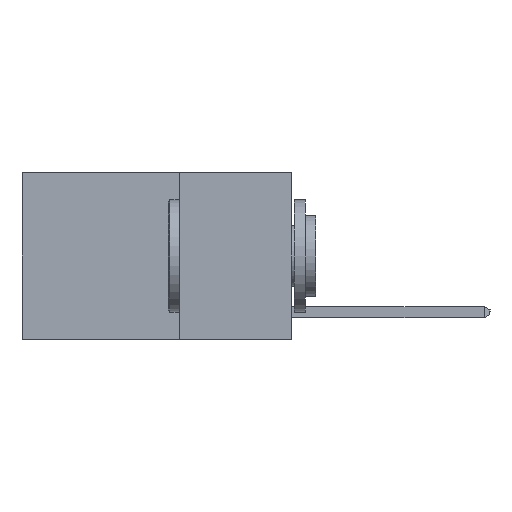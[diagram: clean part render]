
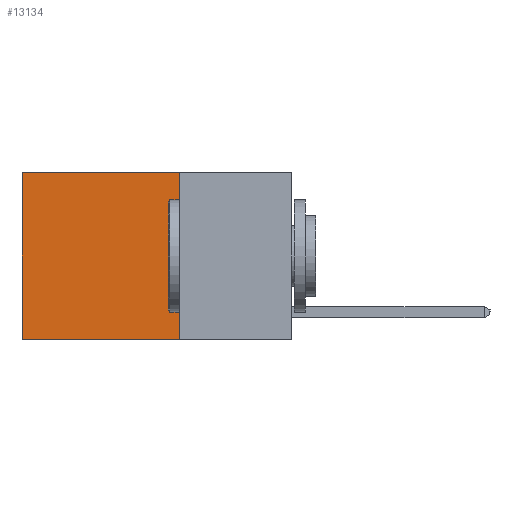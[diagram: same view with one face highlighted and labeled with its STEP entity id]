
A CAD part, left-side view. The second image highlights one B-rep face of the part: STEP entity #13134.
In plain terms, the highlighted planar face has unit normal (-1, 0, 0).
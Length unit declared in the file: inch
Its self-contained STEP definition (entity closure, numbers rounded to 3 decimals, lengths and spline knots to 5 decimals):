
#65 = VERTEX_POINT ( 'NONE', #13806 ) ;
#953 = EDGE_LOOP ( 'NONE', ( #4504, #13131, #11864, #16869 ) ) ;
#1539 = LINE ( 'NONE', #14583, #3955 ) ;
#1749 = DIRECTION ( 'NONE',  ( 0., 0., -1. ) ) ;
#2823 = CARTESIAN_POINT ( 'NONE',  ( 0.2625, 0.25, -0.37 ) ) ;
#3639 = EDGE_CURVE ( 'NONE', #15118, #11644, #1539, .T. ) ;
#3955 = VECTOR ( 'NONE', #12129, 39.37008 ) ;
#4504 = ORIENTED_EDGE ( 'NONE', *, *, #5392, .T. ) ;
#4522 = CARTESIAN_POINT ( 'NONE',  ( 0.2625, 0.25, 0. ) ) ;
#5011 = LINE ( 'NONE', #13721, #15340 ) ;
#5173 = DIRECTION ( 'NONE',  ( 1., 0., 0. ) ) ;
#5254 = VECTOR ( 'NONE', #9857, 39.37008 ) ;
#5392 = EDGE_CURVE ( 'NONE', #7004, #11644, #5011, .T. ) ;
#5666 = LINE ( 'NONE', #16189, #5254 ) ;
#5911 = DIRECTION ( 'NONE',  ( 0., 0., -1. ) ) ;
#7004 = VERTEX_POINT ( 'NONE', #12870 ) ;
#7729 = PLANE ( 'NONE',  #8940 ) ;
#8874 = LINE ( 'NONE', #4522, #11977 ) ;
#8940 = AXIS2_PLACEMENT_3D ( 'NONE', #11705, #5173, #14250 ) ;
#9857 = DIRECTION ( 'NONE',  ( 0., 1., 0. ) ) ;
#11644 = VERTEX_POINT ( 'NONE', #14769 ) ;
#11674 = EDGE_CURVE ( 'NONE', #65, #15118, #8874, .T. ) ;
#11705 = CARTESIAN_POINT ( 'NONE',  ( 0.2625, 0.25, 0. ) ) ;
#11864 = ORIENTED_EDGE ( 'NONE', *, *, #11674, .F. ) ;
#11977 = VECTOR ( 'NONE', #1749, 39.37008 ) ;
#12129 = DIRECTION ( 'NONE',  ( 0., 1., 0. ) ) ;
#12870 = CARTESIAN_POINT ( 'NONE',  ( 0.2625, 0.6, 0. ) ) ;
#13131 = ORIENTED_EDGE ( 'NONE', *, *, #3639, .F. ) ;
#13134 = ADVANCED_FACE ( 'NONE', ( #13907 ), #7729, .F. ) ;
#13721 = CARTESIAN_POINT ( 'NONE',  ( 0.2625, 0.6, 0. ) ) ;
#13806 = CARTESIAN_POINT ( 'NONE',  ( 0.2625, 0.25, 0. ) ) ;
#13907 = FACE_OUTER_BOUND ( 'NONE', #953, .T. ) ;
#14250 = DIRECTION ( 'NONE',  ( 0., 0., -1. ) ) ;
#14583 = CARTESIAN_POINT ( 'NONE',  ( 0.2625, 0.25, -0.37 ) ) ;
#14769 = CARTESIAN_POINT ( 'NONE',  ( 0.2625, 0.6, -0.37 ) ) ;
#15118 = VERTEX_POINT ( 'NONE', #2823 ) ;
#15340 = VECTOR ( 'NONE', #5911, 39.37008 ) ;
#16188 = EDGE_CURVE ( 'NONE', #65, #7004, #5666, .T. ) ;
#16189 = CARTESIAN_POINT ( 'NONE',  ( 0.2625, 0.25, 0. ) ) ;
#16869 = ORIENTED_EDGE ( 'NONE', *, *, #16188, .T. ) ;
